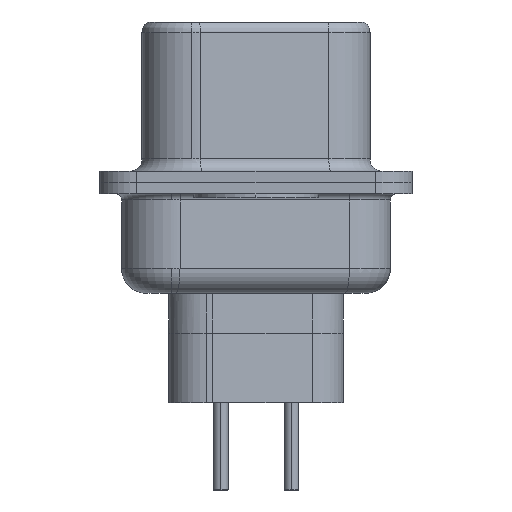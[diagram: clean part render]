
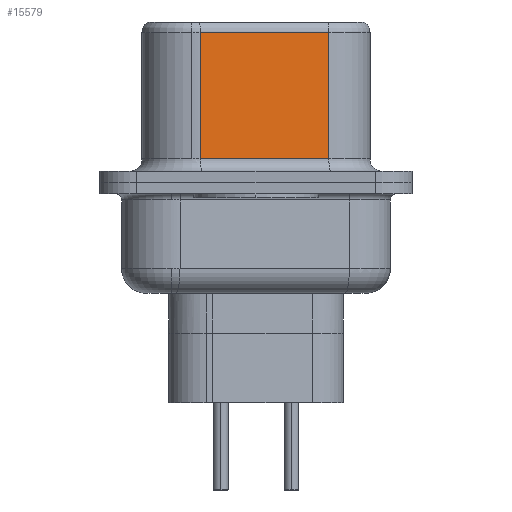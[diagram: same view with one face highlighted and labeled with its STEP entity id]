
A CAD part, left-side view. The second image highlights one B-rep face of the part: STEP entity #15579.
In plain terms, the highlighted planar face has unit normal (-0.985, -0.174, 0).
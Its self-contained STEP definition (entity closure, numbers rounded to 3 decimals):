
#404 = DIRECTION ( 'NONE',  ( 0.985, 0.174, 0. ) ) ;
#1653 = EDGE_CURVE ( 'NONE', #1848, #18036, #1960, .T. ) ;
#1848 = VERTEX_POINT ( 'NONE', #11306 ) ;
#1960 = LINE ( 'NONE', #10323, #5291 ) ;
#2410 = EDGE_CURVE ( 'NONE', #18036, #16707, #17337, .T. ) ;
#2795 = ORIENTED_EDGE ( 'NONE', *, *, #10768, .F. ) ;
#2958 = VECTOR ( 'NONE', #21065, 1000. ) ;
#5291 = VECTOR ( 'NONE', #12131, 1000. ) ;
#6698 = CARTESIAN_POINT ( 'NONE',  ( 4.58, -2.927, 6.52 ) ) ;
#6805 = EDGE_CURVE ( 'NONE', #7025, #1848, #7255, .T. ) ;
#7025 = VERTEX_POINT ( 'NONE', #12682 ) ;
#7255 = LINE ( 'NONE', #23004, #2958 ) ;
#9483 = EDGE_LOOP ( 'NONE', ( #2795, #16332, #9734, #12129 ) ) ;
#9734 = ORIENTED_EDGE ( 'NONE', *, *, #1653, .T. ) ;
#10323 = CARTESIAN_POINT ( 'NONE',  ( 3.67, 2.233, 6.52 ) ) ;
#10768 = EDGE_CURVE ( 'NONE', #7025, #16707, #21637, .T. ) ;
#11306 = CARTESIAN_POINT ( 'NONE',  ( 3.67, 2.233, 6.02 ) ) ;
#11535 = CARTESIAN_POINT ( 'NONE',  ( 3.67, 2.233, 0.95 ) ) ;
#11631 = CARTESIAN_POINT ( 'NONE',  ( 4.58, -2.927, 0.95 ) ) ;
#11859 = VECTOR ( 'NONE', #17598, 1000. ) ;
#12129 = ORIENTED_EDGE ( 'NONE', *, *, #2410, .T. ) ;
#12131 = DIRECTION ( 'NONE',  ( 0., 0., -1. ) ) ;
#12623 = PLANE ( 'NONE',  #16313 ) ;
#12682 = CARTESIAN_POINT ( 'NONE',  ( 4.58, -2.927, 6.02 ) ) ;
#13765 = CARTESIAN_POINT ( 'NONE',  ( 4.58, -2.927, 6.52 ) ) ;
#15404 = CARTESIAN_POINT ( 'NONE',  ( 4.58, -2.927, 0.95 ) ) ;
#15579 = ADVANCED_FACE ( 'NONE', ( #16624 ), #12623, .F. ) ;
#16086 = DIRECTION ( 'NONE',  ( 0., 0., -1. ) ) ;
#16313 = AXIS2_PLACEMENT_3D ( 'NONE', #6698, #404, #24373 ) ;
#16332 = ORIENTED_EDGE ( 'NONE', *, *, #6805, .T. ) ;
#16451 = VECTOR ( 'NONE', #16086, 1000. ) ;
#16624 = FACE_OUTER_BOUND ( 'NONE', #9483, .T. ) ;
#16707 = VERTEX_POINT ( 'NONE', #11631 ) ;
#17337 = LINE ( 'NONE', #15404, #11859 ) ;
#17598 = DIRECTION ( 'NONE',  ( 0.174, -0.985, 0. ) ) ;
#18036 = VERTEX_POINT ( 'NONE', #11535 ) ;
#21065 = DIRECTION ( 'NONE',  ( -0.174, 0.985, 0. ) ) ;
#21637 = LINE ( 'NONE', #13765, #16451 ) ;
#23004 = CARTESIAN_POINT ( 'NONE',  ( 4.58, -2.927, 6.02 ) ) ;
#24373 = DIRECTION ( 'NONE',  ( -0.174, 0.985, 0. ) ) ;
